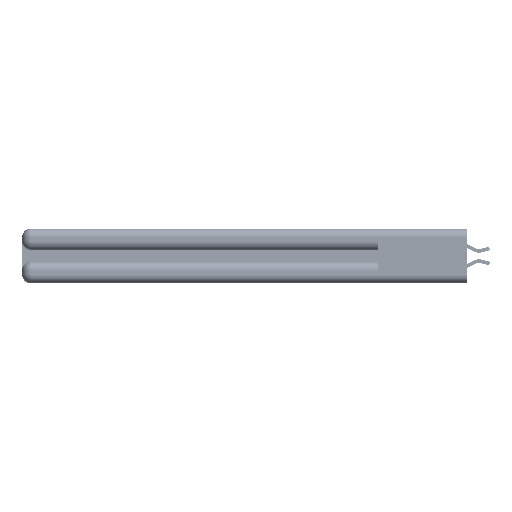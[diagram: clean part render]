
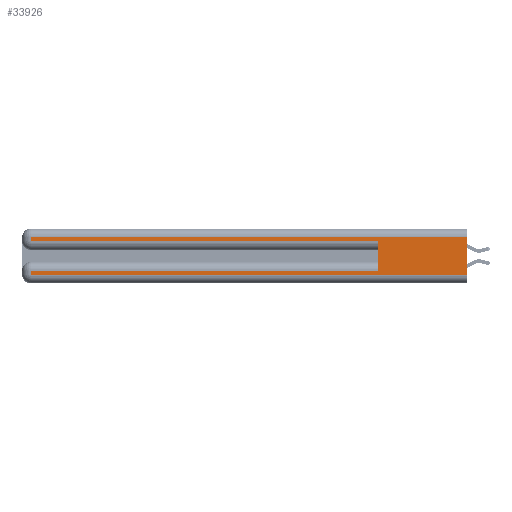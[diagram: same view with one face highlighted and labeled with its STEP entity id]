
A CAD part, left-side view. The second image highlights one B-rep face of the part: STEP entity #33926.
In plain terms, the highlighted planar face has unit normal (-1, 0, 0).
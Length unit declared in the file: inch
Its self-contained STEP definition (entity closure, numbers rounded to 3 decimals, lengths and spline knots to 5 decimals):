
#628 = DIRECTION ( 'NONE',  ( 0., -1., 0. ) ) ;
#677 = LINE ( 'NONE', #39774, #33375 ) ;
#964 = DIRECTION ( 'NONE',  ( 0., 0., -1. ) ) ;
#1303 = CARTESIAN_POINT ( 'NONE',  ( 0., 2.94, 0.37 ) ) ;
#2972 = EDGE_CURVE ( 'NONE', #30232, #49927, #34669, .T. ) ;
#3055 = CARTESIAN_POINT ( 'NONE',  ( 0., 2.94, 0.31 ) ) ;
#4013 = ORIENTED_EDGE ( 'NONE', *, *, #2972, .T. ) ;
#4192 = LINE ( 'NONE', #8838, #16309 ) ;
#4465 = ORIENTED_EDGE ( 'NONE', *, *, #24716, .T. ) ;
#4767 = VECTOR ( 'NONE', #36307, 39.37008 ) ;
#5045 = CARTESIAN_POINT ( 'NONE',  ( 0., 0., 0.31 ) ) ;
#5520 = EDGE_CURVE ( 'NONE', #37749, #33781, #4192, .T. ) ;
#5695 = CARTESIAN_POINT ( 'NONE',  ( 0., 0., 0.06 ) ) ;
#6065 = EDGE_CURVE ( 'NONE', #48083, #49927, #13863, .T. ) ;
#8838 = CARTESIAN_POINT ( 'NONE',  ( 0., 0., 0.37 ) ) ;
#8952 = CARTESIAN_POINT ( 'NONE',  ( 0., 0.6, 0.085 ) ) ;
#9617 = DIRECTION ( 'NONE',  ( 0., 0., -1. ) ) ;
#10916 = DIRECTION ( 'NONE',  ( 0., 1., 0. ) ) ;
#10975 = LINE ( 'NONE', #18549, #30355 ) ;
#11089 = VECTOR ( 'NONE', #628, 39.37008 ) ;
#12687 = AXIS2_PLACEMENT_3D ( 'NONE', #40330, #13462, #39820 ) ;
#13025 = LINE ( 'NONE', #24803, #37225 ) ;
#13462 = DIRECTION ( 'NONE',  ( 1., 0., 0. ) ) ;
#13863 = LINE ( 'NONE', #39853, #4767 ) ;
#13906 = VERTEX_POINT ( 'NONE', #38051 ) ;
#15690 = VERTEX_POINT ( 'NONE', #3055 ) ;
#16309 = VECTOR ( 'NONE', #44493, 39.37008 ) ;
#18549 = CARTESIAN_POINT ( 'NONE',  ( 0., 0., 0.31 ) ) ;
#18677 = VECTOR ( 'NONE', #964, 39.37008 ) ;
#19577 = VECTOR ( 'NONE', #47761, 39.37008 ) ;
#20768 = PLANE ( 'NONE',  #12687 ) ;
#24345 = CARTESIAN_POINT ( 'NONE',  ( 0., 2.94, 0.085 ) ) ;
#24716 = EDGE_CURVE ( 'NONE', #48083, #25099, #677, .T. ) ;
#24803 = CARTESIAN_POINT ( 'NONE',  ( 0., 2.94, 0.37 ) ) ;
#25099 = VERTEX_POINT ( 'NONE', #24345 ) ;
#25437 = ORIENTED_EDGE ( 'NONE', *, *, #5520, .F. ) ;
#26846 = LINE ( 'NONE', #47590, #19577 ) ;
#29874 = EDGE_CURVE ( 'NONE', #15690, #30232, #31366, .T. ) ;
#30232 = VERTEX_POINT ( 'NONE', #34617 ) ;
#30355 = VECTOR ( 'NONE', #10916, 39.37008 ) ;
#31366 = LINE ( 'NONE', #1303, #18677 ) ;
#32968 = ORIENTED_EDGE ( 'NONE', *, *, #6065, .F. ) ;
#32989 = EDGE_CURVE ( 'NONE', #37749, #15690, #10975, .T. ) ;
#33143 = ORIENTED_EDGE ( 'NONE', *, *, #41744, .T. ) ;
#33375 = VECTOR ( 'NONE', #43696, 39.37008 ) ;
#33781 = VERTEX_POINT ( 'NONE', #5695 ) ;
#33926 = ADVANCED_FACE ( 'NONE', ( #36356 ), #20768, .F. ) ;
#33993 = CARTESIAN_POINT ( 'NONE',  ( 0., 0., 0.285 ) ) ;
#34617 = CARTESIAN_POINT ( 'NONE',  ( 0., 2.94, 0.285 ) ) ;
#34669 = LINE ( 'NONE', #33993, #11089 ) ;
#34994 = EDGE_LOOP ( 'NONE', ( #25437, #41227, #48776, #4013, #32968, #4465, #33143, #44896 ) ) ;
#36307 = DIRECTION ( 'NONE',  ( 0., 0., 1. ) ) ;
#36356 = FACE_OUTER_BOUND ( 'NONE', #34994, .T. ) ;
#37225 = VECTOR ( 'NONE', #9617, 39.37008 ) ;
#37749 = VERTEX_POINT ( 'NONE', #5045 ) ;
#38051 = CARTESIAN_POINT ( 'NONE',  ( 0., 2.94, 0.06 ) ) ;
#39774 = CARTESIAN_POINT ( 'NONE',  ( 0., 0., 0.085 ) ) ;
#39820 = DIRECTION ( 'NONE',  ( 0., 0., -1. ) ) ;
#39853 = CARTESIAN_POINT ( 'NONE',  ( 0., 0.6, 0.145 ) ) ;
#40330 = CARTESIAN_POINT ( 'NONE',  ( 0., 0., 0.37 ) ) ;
#41227 = ORIENTED_EDGE ( 'NONE', *, *, #32989, .T. ) ;
#41744 = EDGE_CURVE ( 'NONE', #25099, #13906, #13025, .T. ) ;
#43357 = CARTESIAN_POINT ( 'NONE',  ( 0., 0.6, 0.285 ) ) ;
#43696 = DIRECTION ( 'NONE',  ( 0., 1., 0. ) ) ;
#44493 = DIRECTION ( 'NONE',  ( 0., 0., -1. ) ) ;
#44896 = ORIENTED_EDGE ( 'NONE', *, *, #49537, .T. ) ;
#47590 = CARTESIAN_POINT ( 'NONE',  ( 0., 0., 0.06 ) ) ;
#47761 = DIRECTION ( 'NONE',  ( 0., -1., 0. ) ) ;
#48083 = VERTEX_POINT ( 'NONE', #8952 ) ;
#48776 = ORIENTED_EDGE ( 'NONE', *, *, #29874, .T. ) ;
#49537 = EDGE_CURVE ( 'NONE', #13906, #33781, #26846, .T. ) ;
#49927 = VERTEX_POINT ( 'NONE', #43357 ) ;
